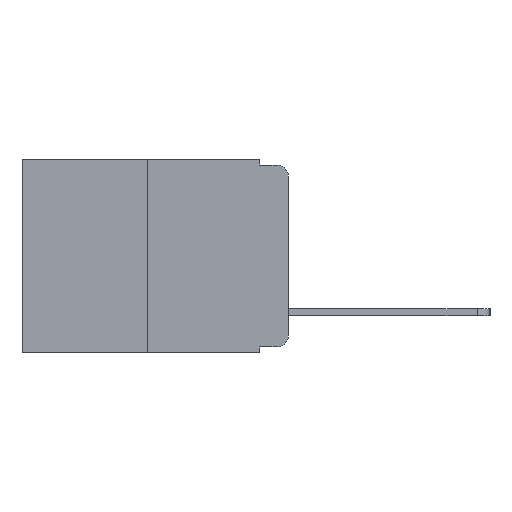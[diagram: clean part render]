
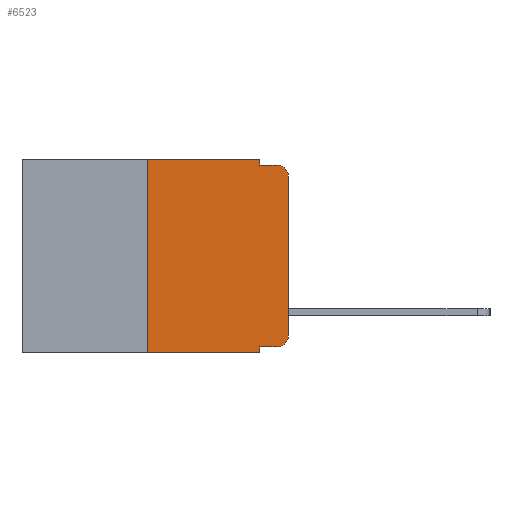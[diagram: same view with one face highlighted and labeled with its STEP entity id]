
A CAD part, left-side view. The second image highlights one B-rep face of the part: STEP entity #6523.
In plain terms, the highlighted planar face has unit normal (-1, 0, 0).
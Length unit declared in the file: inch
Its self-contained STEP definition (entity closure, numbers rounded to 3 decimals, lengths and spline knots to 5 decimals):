
#247 = CIRCLE ( 'NONE', #12202, 0.02 ) ;
#276 = VERTEX_POINT ( 'NONE', #17493 ) ;
#350 = LINE ( 'NONE', #5128, #7691 ) ;
#438 = EDGE_CURVE ( 'NONE', #14400, #8225, #5781, .T. ) ;
#534 = DIRECTION ( 'NONE',  ( 0., -1., 0. ) ) ;
#707 = ORIENTED_EDGE ( 'NONE', *, *, #15155, .T. ) ;
#809 = DIRECTION ( 'NONE',  ( 0., 0., -1. ) ) ;
#857 = EDGE_CURVE ( 'NONE', #4353, #276, #17607, .T. ) ;
#1027 = DIRECTION ( 'NONE',  ( 1., 0., 0. ) ) ;
#1234 = EDGE_CURVE ( 'NONE', #14195, #10215, #247, .T. ) ;
#1409 = VECTOR ( 'NONE', #11386, 39.37008 ) ;
#1795 = DIRECTION ( 'NONE',  ( 0., -1., 0. ) ) ;
#1841 = EDGE_CURVE ( 'NONE', #4353, #11854, #8714, .T. ) ;
#2359 = CARTESIAN_POINT ( 'NONE',  ( 0., 0.25, 0. ) ) ;
#2515 = DIRECTION ( 'NONE',  ( 0., 0., -1. ) ) ;
#2822 = EDGE_CURVE ( 'NONE', #11854, #17908, #11600, .T. ) ;
#3171 = EDGE_CURVE ( 'NONE', #6542, #10215, #9588, .T. ) ;
#3236 = DIRECTION ( 'NONE',  ( -1., 0., 0. ) ) ;
#3510 = CARTESIAN_POINT ( 'NONE',  ( 0., 0.051, 0. ) ) ;
#3895 = DIRECTION ( 'NONE',  ( -1., 0., 0. ) ) ;
#4353 = VERTEX_POINT ( 'NONE', #13351 ) ;
#4774 = CARTESIAN_POINT ( 'NONE',  ( 0., 0.25, -0.343 ) ) ;
#4802 = ORIENTED_EDGE ( 'NONE', *, *, #8087, .F. ) ;
#4847 = DIRECTION ( 'NONE',  ( 0., -1., 0. ) ) ;
#4859 = VECTOR ( 'NONE', #4847, 39.37008 ) ;
#5048 = LINE ( 'NONE', #3510, #16088 ) ;
#5116 = EDGE_CURVE ( 'NONE', #8225, #6542, #5048, .T. ) ;
#5128 = CARTESIAN_POINT ( 'NONE',  ( 0., 0., 0. ) ) ;
#5602 = CARTESIAN_POINT ( 'NONE',  ( 0., 0.051, 0. ) ) ;
#5781 = LINE ( 'NONE', #14940, #4859 ) ;
#6310 = DIRECTION ( 'NONE',  ( 0., 0., -1. ) ) ;
#6314 = CARTESIAN_POINT ( 'NONE',  ( 0., 0.25, 0. ) ) ;
#6523 = ADVANCED_FACE ( 'NONE', ( #11378 ), #14017, .F. ) ;
#6542 = VERTEX_POINT ( 'NONE', #8380 ) ;
#7539 = CARTESIAN_POINT ( 'NONE',  ( 0., 0.02, -0.01 ) ) ;
#7691 = VECTOR ( 'NONE', #16625, 39.37008 ) ;
#8087 = EDGE_CURVE ( 'NONE', #10294, #14400, #18348, .T. ) ;
#8151 = AXIS2_PLACEMENT_3D ( 'NONE', #12575, #3895, #14034 ) ;
#8225 = VERTEX_POINT ( 'NONE', #5602 ) ;
#8235 = DIRECTION ( 'NONE',  ( 0., 0., 1. ) ) ;
#8380 = CARTESIAN_POINT ( 'NONE',  ( 0., 0.051, -0.01 ) ) ;
#8430 = ORIENTED_EDGE ( 'NONE', *, *, #857, .F. ) ;
#8714 = LINE ( 'NONE', #15298, #1409 ) ;
#8880 = CARTESIAN_POINT ( 'NONE',  ( 0., 0.02, -0.333 ) ) ;
#9588 = LINE ( 'NONE', #11944, #13366 ) ;
#10215 = VERTEX_POINT ( 'NONE', #7539 ) ;
#10294 = VERTEX_POINT ( 'NONE', #4774 ) ;
#10883 = VECTOR ( 'NONE', #8235, 39.37008 ) ;
#11215 = DIRECTION ( 'NONE',  ( 0., 0., -1. ) ) ;
#11378 = FACE_OUTER_BOUND ( 'NONE', #11937, .T. ) ;
#11386 = DIRECTION ( 'NONE',  ( 0., -1., 0. ) ) ;
#11600 = CIRCLE ( 'NONE', #8151, 0.02 ) ;
#11854 = VERTEX_POINT ( 'NONE', #8880 ) ;
#11937 = EDGE_LOOP ( 'NONE', ( #707, #16900, #16799, #17421, #16159, #4802, #13094, #8430, #12576, #15376 ) ) ;
#11944 = CARTESIAN_POINT ( 'NONE',  ( 0., 0.051, -0.01 ) ) ;
#12070 = EDGE_CURVE ( 'NONE', #10294, #276, #16989, .T. ) ;
#12202 = AXIS2_PLACEMENT_3D ( 'NONE', #17120, #3236, #2515 ) ;
#12575 = CARTESIAN_POINT ( 'NONE',  ( 0., 0.02, -0.313 ) ) ;
#12576 = ORIENTED_EDGE ( 'NONE', *, *, #1841, .T. ) ;
#13094 = ORIENTED_EDGE ( 'NONE', *, *, #12070, .T. ) ;
#13351 = CARTESIAN_POINT ( 'NONE',  ( 0., 0.051, -0.333 ) ) ;
#13366 = VECTOR ( 'NONE', #1795, 39.37008 ) ;
#13906 = VECTOR ( 'NONE', #809, 39.37008 ) ;
#14017 = PLANE ( 'NONE',  #15733 ) ;
#14034 = DIRECTION ( 'NONE',  ( 0., 0., -1. ) ) ;
#14195 = VERTEX_POINT ( 'NONE', #18656 ) ;
#14400 = VERTEX_POINT ( 'NONE', #6314 ) ;
#14759 = CARTESIAN_POINT ( 'NONE',  ( 0., 0.051, 0. ) ) ;
#14940 = CARTESIAN_POINT ( 'NONE',  ( 0., 0.473, 0. ) ) ;
#14976 = CARTESIAN_POINT ( 'NONE',  ( 0., 0.473, -0.343 ) ) ;
#15155 = EDGE_CURVE ( 'NONE', #17908, #14195, #350, .T. ) ;
#15298 = CARTESIAN_POINT ( 'NONE',  ( 0., 0.051, -0.333 ) ) ;
#15376 = ORIENTED_EDGE ( 'NONE', *, *, #2822, .T. ) ;
#15733 = AXIS2_PLACEMENT_3D ( 'NONE', #18218, #1027, #11215 ) ;
#16088 = VECTOR ( 'NONE', #6310, 39.37008 ) ;
#16159 = ORIENTED_EDGE ( 'NONE', *, *, #438, .F. ) ;
#16552 = VECTOR ( 'NONE', #534, 39.37008 ) ;
#16625 = DIRECTION ( 'NONE',  ( 0., 0., 1. ) ) ;
#16799 = ORIENTED_EDGE ( 'NONE', *, *, #3171, .F. ) ;
#16900 = ORIENTED_EDGE ( 'NONE', *, *, #1234, .T. ) ;
#16989 = LINE ( 'NONE', #14976, #16552 ) ;
#17120 = CARTESIAN_POINT ( 'NONE',  ( 0., 0.02, -0.03 ) ) ;
#17421 = ORIENTED_EDGE ( 'NONE', *, *, #5116, .F. ) ;
#17493 = CARTESIAN_POINT ( 'NONE',  ( 0., 0.051, -0.343 ) ) ;
#17499 = CARTESIAN_POINT ( 'NONE',  ( 0., 0., -0.313 ) ) ;
#17607 = LINE ( 'NONE', #14759, #13906 ) ;
#17908 = VERTEX_POINT ( 'NONE', #17499 ) ;
#18218 = CARTESIAN_POINT ( 'NONE',  ( 0., 0.473, 0. ) ) ;
#18348 = LINE ( 'NONE', #2359, #10883 ) ;
#18656 = CARTESIAN_POINT ( 'NONE',  ( 0., 0., -0.03 ) ) ;
